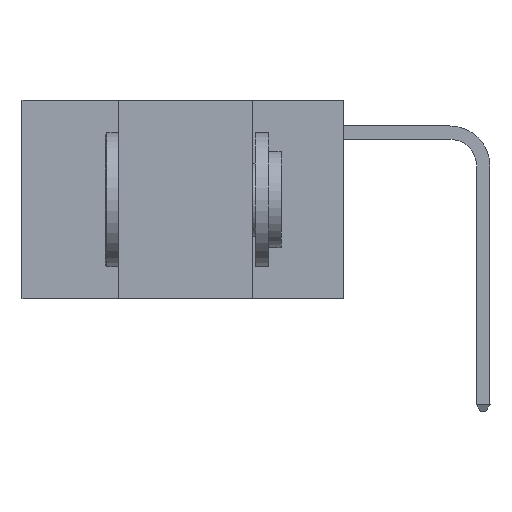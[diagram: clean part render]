
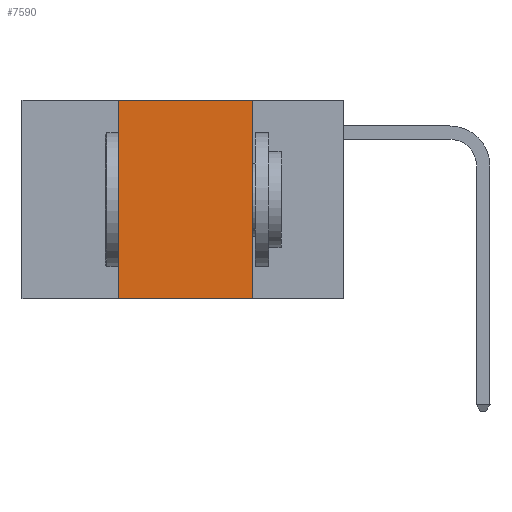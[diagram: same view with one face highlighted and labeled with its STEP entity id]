
A CAD part, left-side view. The second image highlights one B-rep face of the part: STEP entity #7590.
In plain terms, the highlighted planar face has unit normal (-1, 0, 0).
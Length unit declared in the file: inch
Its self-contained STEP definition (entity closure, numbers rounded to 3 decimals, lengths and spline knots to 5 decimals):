
#423 = CARTESIAN_POINT ( 'NONE',  ( 0., 0.42, -0.37 ) ) ;
#1382 = VECTOR ( 'NONE', #9249, 39.37008 ) ;
#2202 = DIRECTION ( 'NONE',  ( 0., 0., -1. ) ) ;
#2325 = EDGE_LOOP ( 'NONE', ( #2743, #12758, #9682, #7671 ) ) ;
#2457 = VECTOR ( 'NONE', #4175, 39.37008 ) ;
#2743 = ORIENTED_EDGE ( 'NONE', *, *, #4583, .F. ) ;
#2826 = CARTESIAN_POINT ( 'NONE',  ( 0., 0.42, 0. ) ) ;
#3181 = LINE ( 'NONE', #7169, #6307 ) ;
#3336 = CARTESIAN_POINT ( 'NONE',  ( 0., 0.17, 0. ) ) ;
#4175 = DIRECTION ( 'NONE',  ( 0., 0., 1. ) ) ;
#4234 = CARTESIAN_POINT ( 'NONE',  ( 0., 0.6, 0. ) ) ;
#4583 = EDGE_CURVE ( 'NONE', #5802, #7562, #10235, .T. ) ;
#4667 = CARTESIAN_POINT ( 'NONE',  ( 0., 0.6, -0.37 ) ) ;
#5802 = VERTEX_POINT ( 'NONE', #3336 ) ;
#6307 = VECTOR ( 'NONE', #9142, 39.37008 ) ;
#6815 = EDGE_CURVE ( 'NONE', #10620, #7562, #11899, .T. ) ;
#7169 = CARTESIAN_POINT ( 'NONE',  ( 0., 0.6, 0. ) ) ;
#7227 = PLANE ( 'NONE',  #10230 ) ;
#7562 = VERTEX_POINT ( 'NONE', #9063 ) ;
#7590 = ADVANCED_FACE ( 'NONE', ( #12249 ), #7227, .F. ) ;
#7671 = ORIENTED_EDGE ( 'NONE', *, *, #6815, .T. ) ;
#7893 = CARTESIAN_POINT ( 'NONE',  ( 0., 0.42, 0. ) ) ;
#8771 = DIRECTION ( 'NONE',  ( 0., -1., 0. ) ) ;
#9063 = CARTESIAN_POINT ( 'NONE',  ( 0., 0.17, -0.37 ) ) ;
#9142 = DIRECTION ( 'NONE',  ( 0., -1., 0. ) ) ;
#9249 = DIRECTION ( 'NONE',  ( 0., 0., -1. ) ) ;
#9682 = ORIENTED_EDGE ( 'NONE', *, *, #11098, .F. ) ;
#10230 = AXIS2_PLACEMENT_3D ( 'NONE', #4234, #11390, #2202 ) ;
#10235 = LINE ( 'NONE', #12441, #1382 ) ;
#10620 = VERTEX_POINT ( 'NONE', #423 ) ;
#11098 = EDGE_CURVE ( 'NONE', #10620, #12978, #13133, .T. ) ;
#11390 = DIRECTION ( 'NONE',  ( 1., 0., 0. ) ) ;
#11899 = LINE ( 'NONE', #4667, #12470 ) ;
#12249 = FACE_OUTER_BOUND ( 'NONE', #2325, .T. ) ;
#12441 = CARTESIAN_POINT ( 'NONE',  ( 0., 0.17, 0. ) ) ;
#12470 = VECTOR ( 'NONE', #8771, 39.37008 ) ;
#12673 = EDGE_CURVE ( 'NONE', #12978, #5802, #3181, .T. ) ;
#12758 = ORIENTED_EDGE ( 'NONE', *, *, #12673, .F. ) ;
#12978 = VERTEX_POINT ( 'NONE', #7893 ) ;
#13133 = LINE ( 'NONE', #2826, #2457 ) ;
